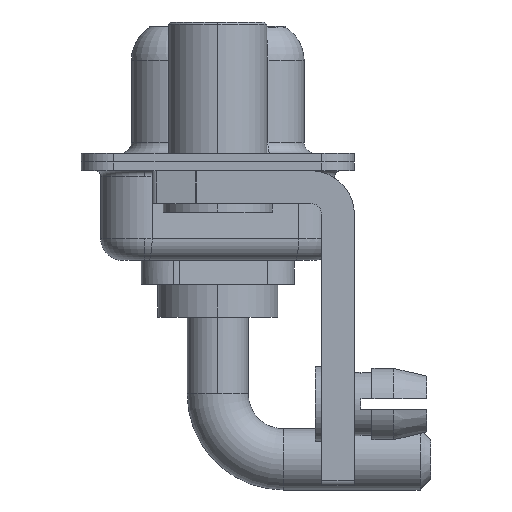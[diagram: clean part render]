
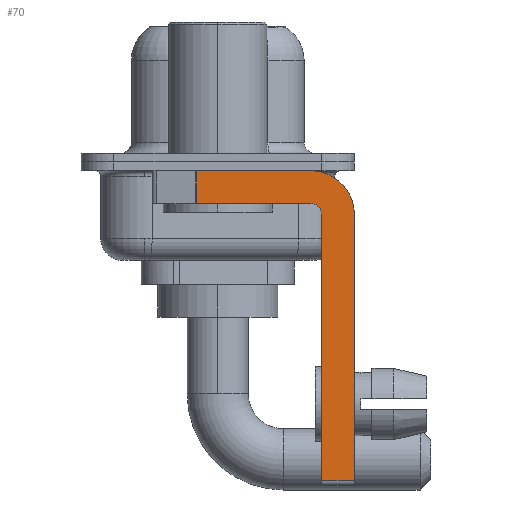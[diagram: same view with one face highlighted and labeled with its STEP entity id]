
A CAD part, left-side view. The second image highlights one B-rep face of the part: STEP entity #70.
In plain terms, the highlighted planar face has unit normal (-1, 0, 0).
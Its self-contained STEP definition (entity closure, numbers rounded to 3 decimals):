
#70 = ADVANCED_FACE ( 'NONE', ( #1647 ), #12779, .F. ) ;
#268 = ORIENTED_EDGE ( 'NONE', *, *, #10100, .F. ) ;
#308 = EDGE_LOOP ( 'NONE', ( #4122, #3958, #4389, #268, #8476, #10654, #6134, #3245 ) ) ;
#518 = DIRECTION ( 'NONE',  ( 0., 0., 1. ) ) ;
#689 = CARTESIAN_POINT ( 'NONE',  ( -2.9, 0.978, -1.9 ) ) ;
#817 = DIRECTION ( 'NONE',  ( -1., 0., 0. ) ) ;
#857 = AXIS2_PLACEMENT_3D ( 'NONE', #1478, #817, #12374 ) ;
#956 = AXIS2_PLACEMENT_3D ( 'NONE', #14923, #6497, #6651 ) ;
#1013 = CARTESIAN_POINT ( 'NONE',  ( -2.9, 3., -0.4 ) ) ;
#1056 = VERTEX_POINT ( 'NONE', #1361 ) ;
#1361 = CARTESIAN_POINT ( 'NONE',  ( -2.9, -4.75, -2.4 ) ) ;
#1478 = CARTESIAN_POINT ( 'NONE',  ( -2.9, -4.25, -2.4 ) ) ;
#1647 = FACE_OUTER_BOUND ( 'NONE', #308, .T. ) ;
#1690 = CARTESIAN_POINT ( 'NONE',  ( -2.9, -4.25, -14.55 ) ) ;
#1777 = EDGE_CURVE ( 'NONE', #2593, #13135, #4222, .T. ) ;
#1987 = VECTOR ( 'NONE', #518, 1000. ) ;
#2118 = CIRCLE ( 'NONE', #857, 0.5 ) ;
#2564 = CARTESIAN_POINT ( 'NONE',  ( -2.9, -6.25, -2.4 ) ) ;
#2593 = VERTEX_POINT ( 'NONE', #5034 ) ;
#2642 = DIRECTION ( 'NONE',  ( 0., 1., 0. ) ) ;
#2652 = EDGE_CURVE ( 'NONE', #2593, #1056, #5589, .T. ) ;
#2693 = DIRECTION ( 'NONE',  ( 0., 0., -1. ) ) ;
#3077 = EDGE_CURVE ( 'NONE', #6080, #14040, #7804, .T. ) ;
#3245 = ORIENTED_EDGE ( 'NONE', *, *, #12186, .F. ) ;
#3940 = EDGE_CURVE ( 'NONE', #8576, #13135, #12570, .T. ) ;
#3958 = ORIENTED_EDGE ( 'NONE', *, *, #8278, .T. ) ;
#4122 = ORIENTED_EDGE ( 'NONE', *, *, #3077, .F. ) ;
#4222 = LINE ( 'NONE', #1690, #12121 ) ;
#4389 = ORIENTED_EDGE ( 'NONE', *, *, #5723, .F. ) ;
#4495 = DIRECTION ( 'NONE',  ( 1., 0., 0. ) ) ;
#4727 = DIRECTION ( 'NONE',  ( 0., 0., -1. ) ) ;
#4879 = CARTESIAN_POINT ( 'NONE',  ( -2.9, -4.25, -1.9 ) ) ;
#5034 = CARTESIAN_POINT ( 'NONE',  ( -2.9, -4.75, -14.55 ) ) ;
#5531 = DIRECTION ( 'NONE',  ( 0., 0., -1. ) ) ;
#5589 = LINE ( 'NONE', #10367, #1987 ) ;
#5626 = VERTEX_POINT ( 'NONE', #13140 ) ;
#5723 = EDGE_CURVE ( 'NONE', #6885, #5626, #13376, .T. ) ;
#5812 = CARTESIAN_POINT ( 'NONE',  ( -2.9, 0.978, -0.4 ) ) ;
#6080 = VERTEX_POINT ( 'NONE', #5812 ) ;
#6134 = ORIENTED_EDGE ( 'NONE', *, *, #3940, .F. ) ;
#6177 = VECTOR ( 'NONE', #12819, 1000. ) ;
#6497 = DIRECTION ( 'NONE',  ( 1., 0., 0. ) ) ;
#6651 = DIRECTION ( 'NONE',  ( 0., 0., -1. ) ) ;
#6885 = VERTEX_POINT ( 'NONE', #4879 ) ;
#7110 = CARTESIAN_POINT ( 'NONE',  ( -2.9, -4.25, -0.4 ) ) ;
#7804 = LINE ( 'NONE', #1013, #6177 ) ;
#8242 = CARTESIAN_POINT ( 'NONE',  ( -2.9, -4.25, -2.4 ) ) ;
#8278 = EDGE_CURVE ( 'NONE', #6080, #5626, #13889, .T. ) ;
#8476 = ORIENTED_EDGE ( 'NONE', *, *, #2652, .F. ) ;
#8576 = VERTEX_POINT ( 'NONE', #2564 ) ;
#8927 = VECTOR ( 'NONE', #2693, 1000. ) ;
#9796 = CARTESIAN_POINT ( 'NONE',  ( -2.9, -4.25, -1.9 ) ) ;
#10100 = EDGE_CURVE ( 'NONE', #1056, #6885, #2118, .T. ) ;
#10367 = CARTESIAN_POINT ( 'NONE',  ( -2.9, -4.75, -14.8 ) ) ;
#10654 = ORIENTED_EDGE ( 'NONE', *, *, #1777, .T. ) ;
#11206 = CARTESIAN_POINT ( 'NONE',  ( -2.9, -6.25, -2.4 ) ) ;
#11317 = VECTOR ( 'NONE', #5531, 1000. ) ;
#11505 = VECTOR ( 'NONE', #2642, 1000. ) ;
#11856 = CARTESIAN_POINT ( 'NONE',  ( -2.9, -6.25, -14.55 ) ) ;
#12121 = VECTOR ( 'NONE', #12595, 1000. ) ;
#12186 = EDGE_CURVE ( 'NONE', #14040, #8576, #14191, .T. ) ;
#12374 = DIRECTION ( 'NONE',  ( 0., 0., 1. ) ) ;
#12570 = LINE ( 'NONE', #11206, #8927 ) ;
#12595 = DIRECTION ( 'NONE',  ( 0., -1., 0. ) ) ;
#12779 = PLANE ( 'NONE',  #956 ) ;
#12819 = DIRECTION ( 'NONE',  ( 0., -1., 0. ) ) ;
#13135 = VERTEX_POINT ( 'NONE', #11856 ) ;
#13140 = CARTESIAN_POINT ( 'NONE',  ( -2.9, 0.978, -1.9 ) ) ;
#13376 = LINE ( 'NONE', #9796, #11505 ) ;
#13889 = LINE ( 'NONE', #689, #11317 ) ;
#14040 = VERTEX_POINT ( 'NONE', #7110 ) ;
#14191 = CIRCLE ( 'NONE', #14954, 2. ) ;
#14923 = CARTESIAN_POINT ( 'NONE',  ( -2.9, -4.25, -2.4 ) ) ;
#14954 = AXIS2_PLACEMENT_3D ( 'NONE', #8242, #4495, #4727 ) ;
